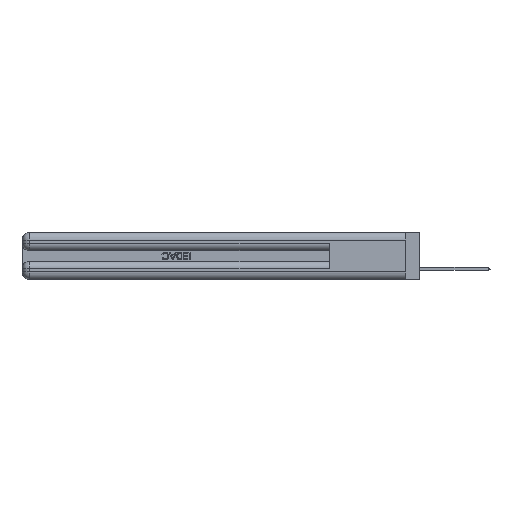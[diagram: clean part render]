
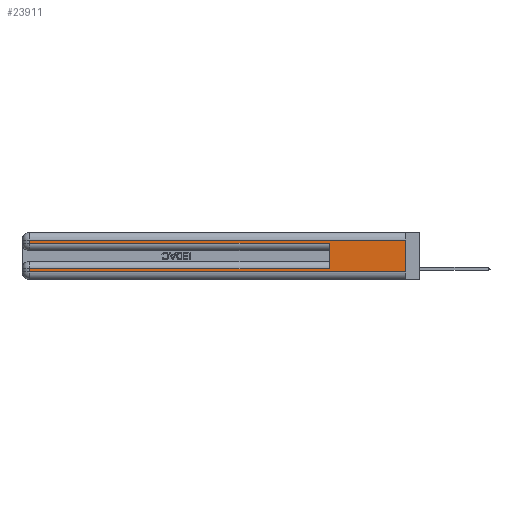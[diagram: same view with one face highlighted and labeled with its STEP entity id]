
A CAD part, left-side view. The second image highlights one B-rep face of the part: STEP entity #23911.
In plain terms, the highlighted planar face has unit normal (-1, 0, 0).
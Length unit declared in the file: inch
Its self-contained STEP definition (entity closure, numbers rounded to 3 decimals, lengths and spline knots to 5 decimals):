
#12 = ORIENTED_EDGE ( 'NONE', *, *, #27979, .T. ) ;
#482 = CARTESIAN_POINT ( 'NONE',  ( 0., 2.94, 0.31 ) ) ;
#2455 = VECTOR ( 'NONE', #14434, 39.37008 ) ;
#2542 = CARTESIAN_POINT ( 'NONE',  ( 0., 2.94, 0.37 ) ) ;
#3127 = EDGE_CURVE ( 'NONE', #9874, #29921, #43825, .T. ) ;
#3671 = EDGE_CURVE ( 'NONE', #10368, #29921, #34077, .T. ) ;
#4056 = ORIENTED_EDGE ( 'NONE', *, *, #30520, .T. ) ;
#4622 = DIRECTION ( 'NONE',  ( 0., 0., 1. ) ) ;
#4630 = VECTOR ( 'NONE', #42600, 39.37008 ) ;
#4790 = CARTESIAN_POINT ( 'NONE',  ( 0., 2.94, 0.37 ) ) ;
#5947 = DIRECTION ( 'NONE',  ( 0., 0., -1. ) ) ;
#7050 = VERTEX_POINT ( 'NONE', #35721 ) ;
#7210 = AXIS2_PLACEMENT_3D ( 'NONE', #15381, #25854, #39242 ) ;
#8206 = EDGE_CURVE ( 'NONE', #41192, #7050, #35731, .T. ) ;
#9874 = VERTEX_POINT ( 'NONE', #33220 ) ;
#10330 = EDGE_CURVE ( 'NONE', #14503, #35091, #15778, .T. ) ;
#10368 = VERTEX_POINT ( 'NONE', #32174 ) ;
#10691 = VECTOR ( 'NONE', #4622, 39.37008 ) ;
#11335 = CARTESIAN_POINT ( 'NONE',  ( 0., 0.6, 0.085 ) ) ;
#12629 = ORIENTED_EDGE ( 'NONE', *, *, #10330, .T. ) ;
#13954 = LINE ( 'NONE', #15392, #10691 ) ;
#14344 = EDGE_LOOP ( 'NONE', ( #37080, #12, #4056, #12629, #26301, #14935, #33710, #17203 ) ) ;
#14434 = DIRECTION ( 'NONE',  ( 0., -1., 0. ) ) ;
#14503 = VERTEX_POINT ( 'NONE', #14814 ) ;
#14814 = CARTESIAN_POINT ( 'NONE',  ( 0., 2.94, 0.285 ) ) ;
#14935 = ORIENTED_EDGE ( 'NONE', *, *, #8206, .T. ) ;
#15381 = CARTESIAN_POINT ( 'NONE',  ( 0., 0., 0.37 ) ) ;
#15392 = CARTESIAN_POINT ( 'NONE',  ( 0., 0.6, 0.145 ) ) ;
#15778 = LINE ( 'NONE', #42388, #2455 ) ;
#16921 = VECTOR ( 'NONE', #36375, 39.37008 ) ;
#17203 = ORIENTED_EDGE ( 'NONE', *, *, #3671, .T. ) ;
#20055 = CARTESIAN_POINT ( 'NONE',  ( 0., 0., 0.085 ) ) ;
#20229 = CARTESIAN_POINT ( 'NONE',  ( 0., 0., 0.31 ) ) ;
#20264 = CARTESIAN_POINT ( 'NONE',  ( 0., 0.6, 0.285 ) ) ;
#23478 = DIRECTION ( 'NONE',  ( 0., 1., 0. ) ) ;
#23911 = ADVANCED_FACE ( 'NONE', ( #31236 ), #36092, .F. ) ;
#24584 = VECTOR ( 'NONE', #39741, 39.37008 ) ;
#25854 = DIRECTION ( 'NONE',  ( 1., 0., 0. ) ) ;
#26301 = ORIENTED_EDGE ( 'NONE', *, *, #43979, .F. ) ;
#27608 = VERTEX_POINT ( 'NONE', #482 ) ;
#27829 = LINE ( 'NONE', #20229, #24584 ) ;
#27979 = EDGE_CURVE ( 'NONE', #9874, #27608, #27829, .T. ) ;
#29921 = VERTEX_POINT ( 'NONE', #31259 ) ;
#30520 = EDGE_CURVE ( 'NONE', #27608, #14503, #36809, .T. ) ;
#31236 = FACE_OUTER_BOUND ( 'NONE', #14344, .T. ) ;
#31259 = CARTESIAN_POINT ( 'NONE',  ( 0., 0., 0.06 ) ) ;
#32174 = CARTESIAN_POINT ( 'NONE',  ( 0., 2.94, 0.06 ) ) ;
#32911 = CARTESIAN_POINT ( 'NONE',  ( 0., 0., 0.06 ) ) ;
#33220 = CARTESIAN_POINT ( 'NONE',  ( 0., 0., 0.31 ) ) ;
#33710 = ORIENTED_EDGE ( 'NONE', *, *, #36335, .T. ) ;
#33941 = CARTESIAN_POINT ( 'NONE',  ( 0., 0., 0.37 ) ) ;
#34077 = LINE ( 'NONE', #32911, #16921 ) ;
#35091 = VERTEX_POINT ( 'NONE', #20264 ) ;
#35715 = VECTOR ( 'NONE', #40094, 39.37008 ) ;
#35721 = CARTESIAN_POINT ( 'NONE',  ( 0., 2.94, 0.085 ) ) ;
#35731 = LINE ( 'NONE', #20055, #38956 ) ;
#36092 = PLANE ( 'NONE',  #7210 ) ;
#36335 = EDGE_CURVE ( 'NONE', #7050, #10368, #40409, .T. ) ;
#36375 = DIRECTION ( 'NONE',  ( 0., -1., 0. ) ) ;
#36809 = LINE ( 'NONE', #4790, #4630 ) ;
#37080 = ORIENTED_EDGE ( 'NONE', *, *, #3127, .F. ) ;
#38956 = VECTOR ( 'NONE', #23478, 39.37008 ) ;
#39242 = DIRECTION ( 'NONE',  ( 0., 0., -1. ) ) ;
#39741 = DIRECTION ( 'NONE',  ( 0., 1., 0. ) ) ;
#40094 = DIRECTION ( 'NONE',  ( 0., 0., -1. ) ) ;
#40409 = LINE ( 'NONE', #2542, #40939 ) ;
#40939 = VECTOR ( 'NONE', #5947, 39.37008 ) ;
#41192 = VERTEX_POINT ( 'NONE', #11335 ) ;
#42388 = CARTESIAN_POINT ( 'NONE',  ( 0., 0., 0.285 ) ) ;
#42600 = DIRECTION ( 'NONE',  ( 0., 0., -1. ) ) ;
#43825 = LINE ( 'NONE', #33941, #35715 ) ;
#43979 = EDGE_CURVE ( 'NONE', #41192, #35091, #13954, .T. ) ;
